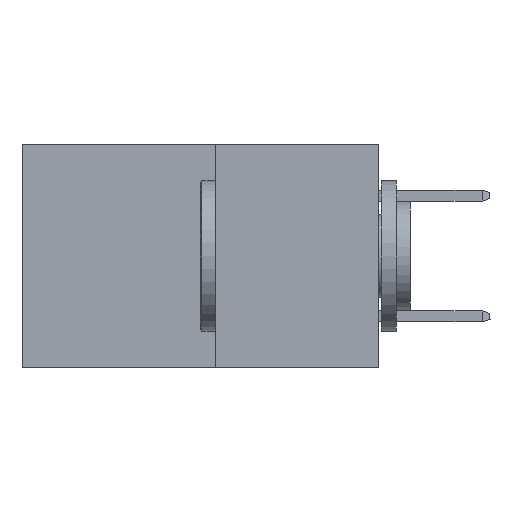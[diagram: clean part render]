
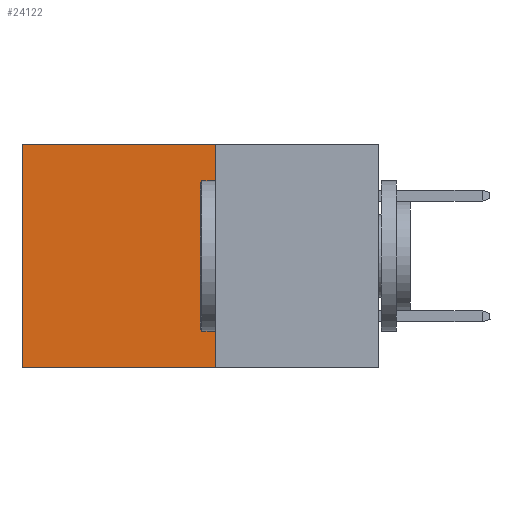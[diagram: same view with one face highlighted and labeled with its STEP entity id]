
A CAD part, left-side view. The second image highlights one B-rep face of the part: STEP entity #24122.
In plain terms, the highlighted planar face has unit normal (-1, 0, 0).
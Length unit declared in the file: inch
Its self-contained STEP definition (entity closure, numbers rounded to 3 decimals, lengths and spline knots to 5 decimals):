
#715 = EDGE_CURVE ( 'NONE', #2437, #20015, #12116, .T. ) ;
#2437 = VERTEX_POINT ( 'NONE', #13373 ) ;
#3210 = EDGE_CURVE ( 'NONE', #20858, #2437, #15655, .T. ) ;
#3411 = CARTESIAN_POINT ( 'NONE',  ( 0.277, 0.27, -0.37 ) ) ;
#5421 = DIRECTION ( 'NONE',  ( 0., 0., -1. ) ) ;
#6257 = CARTESIAN_POINT ( 'NONE',  ( 0.277, 0.27, 0. ) ) ;
#6512 = DIRECTION ( 'NONE',  ( 1., 0., 0. ) ) ;
#6539 = EDGE_CURVE ( 'NONE', #23771, #20015, #11351, .T. ) ;
#6671 = VECTOR ( 'NONE', #10812, 39.37008 ) ;
#7169 = DIRECTION ( 'NONE',  ( 0., 1., 0. ) ) ;
#7526 = ORIENTED_EDGE ( 'NONE', *, *, #3210, .T. ) ;
#7824 = CARTESIAN_POINT ( 'NONE',  ( 0.277, 0.27, 0. ) ) ;
#10184 = VECTOR ( 'NONE', #7169, 39.37008 ) ;
#10812 = DIRECTION ( 'NONE',  ( 0., 0., -1. ) ) ;
#11351 = LINE ( 'NONE', #24021, #16146 ) ;
#11352 = EDGE_LOOP ( 'NONE', ( #23778, #24128, #15235, #7526 ) ) ;
#12116 = LINE ( 'NONE', #12790, #6671 ) ;
#12790 = CARTESIAN_POINT ( 'NONE',  ( 0.277, 0.59, -0.37 ) ) ;
#13373 = CARTESIAN_POINT ( 'NONE',  ( 0.277, 0.59, 0. ) ) ;
#15235 = ORIENTED_EDGE ( 'NONE', *, *, #17705, .F. ) ;
#15598 = CARTESIAN_POINT ( 'NONE',  ( 0.277, 0.27, -0.37 ) ) ;
#15655 = LINE ( 'NONE', #7824, #10184 ) ;
#16146 = VECTOR ( 'NONE', #23221, 39.37008 ) ;
#17705 = EDGE_CURVE ( 'NONE', #20858, #23771, #26255, .T. ) ;
#18776 = PLANE ( 'NONE',  #26363 ) ;
#19931 = FACE_OUTER_BOUND ( 'NONE', #11352, .T. ) ;
#20015 = VERTEX_POINT ( 'NONE', #20352 ) ;
#20352 = CARTESIAN_POINT ( 'NONE',  ( 0.277, 0.59, -0.37 ) ) ;
#20765 = VECTOR ( 'NONE', #5421, 39.37008 ) ;
#20776 = CARTESIAN_POINT ( 'NONE',  ( 0.277, 0.27, -0.37 ) ) ;
#20858 = VERTEX_POINT ( 'NONE', #6257 ) ;
#20872 = DIRECTION ( 'NONE',  ( 0., 0., -1. ) ) ;
#23221 = DIRECTION ( 'NONE',  ( 0., 1., 0. ) ) ;
#23771 = VERTEX_POINT ( 'NONE', #3411 ) ;
#23778 = ORIENTED_EDGE ( 'NONE', *, *, #715, .T. ) ;
#24021 = CARTESIAN_POINT ( 'NONE',  ( 0.277, 0.27, -0.37 ) ) ;
#24122 = ADVANCED_FACE ( 'NONE', ( #19931 ), #18776, .F. ) ;
#24128 = ORIENTED_EDGE ( 'NONE', *, *, #6539, .F. ) ;
#26255 = LINE ( 'NONE', #15598, #20765 ) ;
#26363 = AXIS2_PLACEMENT_3D ( 'NONE', #20776, #6512, #20872 ) ;
